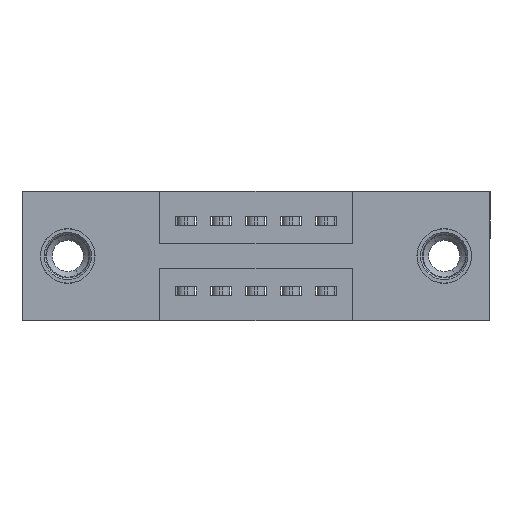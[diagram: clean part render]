
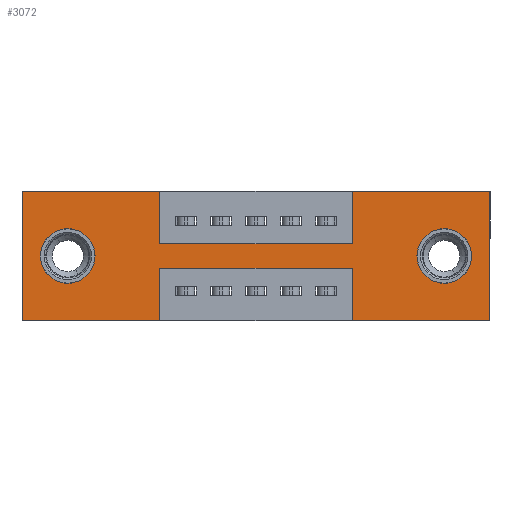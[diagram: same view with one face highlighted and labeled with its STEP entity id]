
A CAD part, front view. The second image highlights one B-rep face of the part: STEP entity #3072.
In plain terms, the highlighted planar face has unit normal (0, -1, 0).
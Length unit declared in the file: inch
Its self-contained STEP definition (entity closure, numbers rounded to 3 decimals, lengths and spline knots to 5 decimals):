
#96 = LINE ( 'NONE', #9319, #3574 ) ;
#143 = EDGE_CURVE ( 'NONE', #10150, #1979, #2910, .T. ) ;
#213 = ORIENTED_EDGE ( 'NONE', *, *, #7213, .F. ) ;
#301 = FACE_BOUND ( 'NONE', #7372, .T. ) ;
#498 = EDGE_CURVE ( 'NONE', #9902, #1487, #895, .T. ) ;
#556 = CARTESIAN_POINT ( 'NONE',  ( 0., 0., 0. ) ) ;
#591 = ORIENTED_EDGE ( 'NONE', *, *, #3108, .F. ) ;
#768 = VECTOR ( 'NONE', #5373, 39.37008 ) ;
#850 = VERTEX_POINT ( 'NONE', #10096 ) ;
#895 = CIRCLE ( 'NONE', #4457, 0.078 ) ;
#907 = EDGE_LOOP ( 'NONE', ( #213, #5333, #10162, #9071, #7268, #8122, #4781, #996, #6854, #9447, #591, #1463 ) ) ;
#972 = FACE_BOUND ( 'NONE', #4320, .T. ) ;
#996 = ORIENTED_EDGE ( 'NONE', *, *, #4130, .F. ) ;
#1199 = DIRECTION ( 'NONE',  ( 0., 1., 0. ) ) ;
#1212 = EDGE_CURVE ( 'NONE', #1487, #9902, #4189, .T. ) ;
#1373 = VECTOR ( 'NONE', #8853, 39.37008 ) ;
#1454 = VERTEX_POINT ( 'NONE', #8207 ) ;
#1463 = ORIENTED_EDGE ( 'NONE', *, *, #2806, .F. ) ;
#1479 = LINE ( 'NONE', #7259, #10905 ) ;
#1487 = VERTEX_POINT ( 'NONE', #8241 ) ;
#1506 = DIRECTION ( 'NONE',  ( 0., 0., -1. ) ) ;
#1596 = ORIENTED_EDGE ( 'NONE', *, *, #1212, .T. ) ;
#1706 = DIRECTION ( 'NONE',  ( -1., 0., 0. ) ) ;
#1806 = LINE ( 'NONE', #3480, #3810 ) ;
#1822 = AXIS2_PLACEMENT_3D ( 'NONE', #2065, #5595, #9722 ) ;
#1827 = DIRECTION ( 'NONE',  ( 0., 1., 0. ) ) ;
#1913 = CARTESIAN_POINT ( 'NONE',  ( 0.13, 0., -0.185 ) ) ;
#1979 = VERTEX_POINT ( 'NONE', #7046 ) ;
#2065 = CARTESIAN_POINT ( 'NONE',  ( 0., 0., -0.37 ) ) ;
#2158 = VECTOR ( 'NONE', #2203, 39.37008 ) ;
#2196 = VERTEX_POINT ( 'NONE', #5744 ) ;
#2203 = DIRECTION ( 'NONE',  ( 0., 0., 1. ) ) ;
#2487 = DIRECTION ( 'NONE',  ( 1., 0., 0. ) ) ;
#2631 = DIRECTION ( 'NONE',  ( 0., 0., -1. ) ) ;
#2753 = EDGE_CURVE ( 'NONE', #850, #6188, #9757, .T. ) ;
#2806 = EDGE_CURVE ( 'NONE', #1454, #3682, #3115, .T. ) ;
#2879 = VECTOR ( 'NONE', #5055, 39.37008 ) ;
#2910 = LINE ( 'NONE', #7072, #768 ) ;
#3071 = VERTEX_POINT ( 'NONE', #9808 ) ;
#3072 = ADVANCED_FACE ( 'NONE', ( #301, #972, #9060 ), #7186, .T. ) ;
#3108 = EDGE_CURVE ( 'NONE', #3682, #4323, #6160, .T. ) ;
#3115 = LINE ( 'NONE', #7601, #3389 ) ;
#3369 = DIRECTION ( 'NONE',  ( 0., 0., -1. ) ) ;
#3389 = VECTOR ( 'NONE', #1706, 39.37008 ) ;
#3458 = EDGE_CURVE ( 'NONE', #6188, #10150, #96, .T. ) ;
#3480 = CARTESIAN_POINT ( 'NONE',  ( 0.9425, 0., -0.37 ) ) ;
#3522 = VECTOR ( 'NONE', #3369, 39.37008 ) ;
#3573 = CARTESIAN_POINT ( 'NONE',  ( 1.335, 0., 0. ) ) ;
#3574 = VECTOR ( 'NONE', #5323, 39.37008 ) ;
#3682 = VERTEX_POINT ( 'NONE', #7394 ) ;
#3779 = VECTOR ( 'NONE', #2487, 39.37008 ) ;
#3810 = VECTOR ( 'NONE', #7577, 39.37008 ) ;
#3902 = CARTESIAN_POINT ( 'NONE',  ( 0.13, 0., -0.185 ) ) ;
#4130 = EDGE_CURVE ( 'NONE', #4729, #6582, #1479, .T. ) ;
#4189 = CIRCLE ( 'NONE', #5458, 0.078 ) ;
#4320 = EDGE_LOOP ( 'NONE', ( #1596, #6176 ) ) ;
#4323 = VERTEX_POINT ( 'NONE', #556 ) ;
#4426 = CARTESIAN_POINT ( 'NONE',  ( 0.3925, 0., -0.22 ) ) ;
#4457 = AXIS2_PLACEMENT_3D ( 'NONE', #3902, #7392, #5715 ) ;
#4674 = LINE ( 'NONE', #7001, #5856 ) ;
#4709 = EDGE_CURVE ( 'NONE', #4323, #3071, #4674, .T. ) ;
#4729 = VERTEX_POINT ( 'NONE', #10400 ) ;
#4781 = ORIENTED_EDGE ( 'NONE', *, *, #6432, .F. ) ;
#4887 = CARTESIAN_POINT ( 'NONE',  ( 0.3925, 0., -0.22 ) ) ;
#5055 = DIRECTION ( 'NONE',  ( 0., 0., -1. ) ) ;
#5259 = LINE ( 'NONE', #7726, #2879 ) ;
#5323 = DIRECTION ( 'NONE',  ( 0., 0., -1. ) ) ;
#5333 = ORIENTED_EDGE ( 'NONE', *, *, #6866, .F. ) ;
#5369 = DIRECTION ( 'NONE',  ( 1., 0., 0. ) ) ;
#5373 = DIRECTION ( 'NONE',  ( -1., 0., 0. ) ) ;
#5458 = AXIS2_PLACEMENT_3D ( 'NONE', #1913, #1199, #7158 ) ;
#5595 = DIRECTION ( 'NONE',  ( 0., -1., 0. ) ) ;
#5625 = CARTESIAN_POINT ( 'NONE',  ( 0., 0., 0. ) ) ;
#5644 = ORIENTED_EDGE ( 'NONE', *, *, #7151, .T. ) ;
#5715 = DIRECTION ( 'NONE',  ( 0., 0., 1. ) ) ;
#5744 = CARTESIAN_POINT ( 'NONE',  ( 1.205, 0., -0.107 ) ) ;
#5856 = VECTOR ( 'NONE', #5369, 39.37008 ) ;
#5879 = CARTESIAN_POINT ( 'NONE',  ( 0.9425, 0., -0.15 ) ) ;
#6160 = LINE ( 'NONE', #5625, #1373 ) ;
#6176 = ORIENTED_EDGE ( 'NONE', *, *, #498, .T. ) ;
#6188 = VERTEX_POINT ( 'NONE', #3573 ) ;
#6432 = EDGE_CURVE ( 'NONE', #6582, #850, #9880, .T. ) ;
#6582 = VERTEX_POINT ( 'NONE', #5879 ) ;
#6854 = ORIENTED_EDGE ( 'NONE', *, *, #8561, .F. ) ;
#6866 = EDGE_CURVE ( 'NONE', #7029, #8291, #8395, .T. ) ;
#6999 = AXIS2_PLACEMENT_3D ( 'NONE', #7695, #1827, #2631 ) ;
#7001 = CARTESIAN_POINT ( 'NONE',  ( 0., 0., 0. ) ) ;
#7003 = CIRCLE ( 'NONE', #9505, 0.078 ) ;
#7029 = VERTEX_POINT ( 'NONE', #10931 ) ;
#7046 = CARTESIAN_POINT ( 'NONE',  ( 0.9425, 0., -0.37 ) ) ;
#7055 = DIRECTION ( 'NONE',  ( -1., 0., 0. ) ) ;
#7072 = CARTESIAN_POINT ( 'NONE',  ( 0., 0., -0.37 ) ) ;
#7151 = EDGE_CURVE ( 'NONE', #7575, #2196, #10965, .T. ) ;
#7158 = DIRECTION ( 'NONE',  ( 0., 0., 1. ) ) ;
#7186 = PLANE ( 'NONE',  #1822 ) ;
#7213 = EDGE_CURVE ( 'NONE', #8291, #1454, #5259, .T. ) ;
#7259 = CARTESIAN_POINT ( 'NONE',  ( 0.3925, 0., -0.15 ) ) ;
#7268 = ORIENTED_EDGE ( 'NONE', *, *, #3458, .F. ) ;
#7350 = CARTESIAN_POINT ( 'NONE',  ( 1.205, 0., -0.263 ) ) ;
#7372 = EDGE_LOOP ( 'NONE', ( #10929, #5644 ) ) ;
#7392 = DIRECTION ( 'NONE',  ( 0., 1., 0. ) ) ;
#7394 = CARTESIAN_POINT ( 'NONE',  ( 0., 0., -0.37 ) ) ;
#7481 = DIRECTION ( 'NONE',  ( 0., 1., 0. ) ) ;
#7575 = VERTEX_POINT ( 'NONE', #7350 ) ;
#7577 = DIRECTION ( 'NONE',  ( 0., 0., 1. ) ) ;
#7601 = CARTESIAN_POINT ( 'NONE',  ( 0., 0., -0.37 ) ) ;
#7695 = CARTESIAN_POINT ( 'NONE',  ( 1.205, 0., -0.185 ) ) ;
#7726 = CARTESIAN_POINT ( 'NONE',  ( 0.3925, 0., -0.37 ) ) ;
#8122 = ORIENTED_EDGE ( 'NONE', *, *, #2753, .F. ) ;
#8207 = CARTESIAN_POINT ( 'NONE',  ( 0.3925, 0., -0.37 ) ) ;
#8241 = CARTESIAN_POINT ( 'NONE',  ( 0.13, 0., -0.107 ) ) ;
#8291 = VERTEX_POINT ( 'NONE', #4887 ) ;
#8323 = CARTESIAN_POINT ( 'NONE',  ( 1.205, 0., -0.185 ) ) ;
#8348 = CARTESIAN_POINT ( 'NONE',  ( 0.3925, 0., 0. ) ) ;
#8361 = CARTESIAN_POINT ( 'NONE',  ( 0., 0., 0. ) ) ;
#8395 = LINE ( 'NONE', #4426, #10022 ) ;
#8478 = CARTESIAN_POINT ( 'NONE',  ( 0.13, 0., -0.263 ) ) ;
#8561 = EDGE_CURVE ( 'NONE', #3071, #4729, #10794, .T. ) ;
#8853 = DIRECTION ( 'NONE',  ( 0., 0., 1. ) ) ;
#9060 = FACE_OUTER_BOUND ( 'NONE', #907, .T. ) ;
#9071 = ORIENTED_EDGE ( 'NONE', *, *, #143, .F. ) ;
#9319 = CARTESIAN_POINT ( 'NONE',  ( 1.335, 0., 0. ) ) ;
#9447 = ORIENTED_EDGE ( 'NONE', *, *, #4709, .F. ) ;
#9505 = AXIS2_PLACEMENT_3D ( 'NONE', #8323, #7481, #1506 ) ;
#9693 = EDGE_CURVE ( 'NONE', #2196, #7575, #7003, .T. ) ;
#9722 = DIRECTION ( 'NONE',  ( 0., 0., -1. ) ) ;
#9747 = DIRECTION ( 'NONE',  ( 1., 0., 0. ) ) ;
#9757 = LINE ( 'NONE', #8361, #3779 ) ;
#9808 = CARTESIAN_POINT ( 'NONE',  ( 0.3925, 0., 0. ) ) ;
#9880 = LINE ( 'NONE', #9943, #2158 ) ;
#9902 = VERTEX_POINT ( 'NONE', #8478 ) ;
#9943 = CARTESIAN_POINT ( 'NONE',  ( 0.9425, 0., 0. ) ) ;
#10022 = VECTOR ( 'NONE', #7055, 39.37008 ) ;
#10096 = CARTESIAN_POINT ( 'NONE',  ( 0.9425, 0., 0. ) ) ;
#10150 = VERTEX_POINT ( 'NONE', #10154 ) ;
#10154 = CARTESIAN_POINT ( 'NONE',  ( 1.335, 0., -0.37 ) ) ;
#10162 = ORIENTED_EDGE ( 'NONE', *, *, #10755, .F. ) ;
#10400 = CARTESIAN_POINT ( 'NONE',  ( 0.3925, 0., -0.15 ) ) ;
#10755 = EDGE_CURVE ( 'NONE', #1979, #7029, #1806, .T. ) ;
#10794 = LINE ( 'NONE', #8348, #3522 ) ;
#10905 = VECTOR ( 'NONE', #9747, 39.37008 ) ;
#10929 = ORIENTED_EDGE ( 'NONE', *, *, #9693, .T. ) ;
#10931 = CARTESIAN_POINT ( 'NONE',  ( 0.9425, 0., -0.22 ) ) ;
#10965 = CIRCLE ( 'NONE', #6999, 0.078 ) ;
